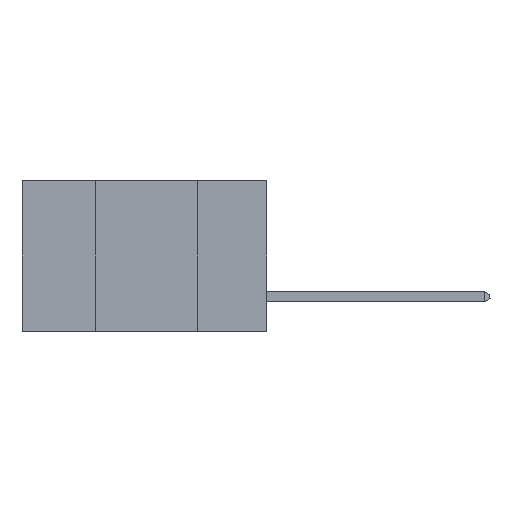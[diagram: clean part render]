
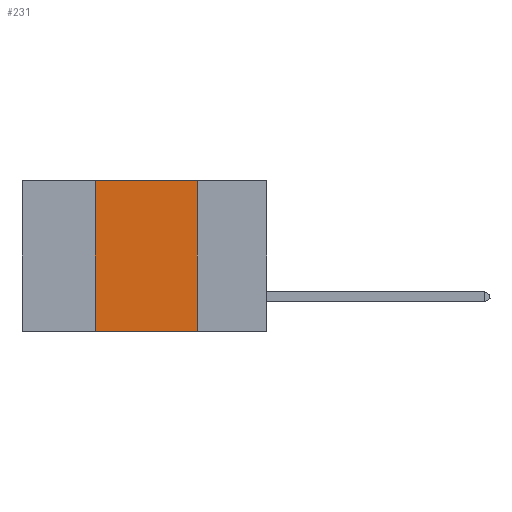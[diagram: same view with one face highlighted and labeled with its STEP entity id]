
A CAD part, left-side view. The second image highlights one B-rep face of the part: STEP entity #231.
In plain terms, the highlighted planar face has unit normal (-1, 0, 0).
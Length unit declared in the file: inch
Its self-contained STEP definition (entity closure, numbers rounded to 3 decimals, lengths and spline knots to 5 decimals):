
#231 = ADVANCED_FACE ( 'NONE', ( #3089 ), #13129, .F. ) ;
#276 = AXIS2_PLACEMENT_3D ( 'NONE', #3503, #13479, #14699 ) ;
#319 = EDGE_LOOP ( 'NONE', ( #8522, #7369, #3352, #14893 ) ) ;
#569 = LINE ( 'NONE', #1168, #6791 ) ;
#681 = CARTESIAN_POINT ( 'NONE',  ( 0., 0.42, -0.37 ) ) ;
#1168 = CARTESIAN_POINT ( 'NONE',  ( 0., 0.42, 0. ) ) ;
#1936 = VECTOR ( 'NONE', #8926, 39.37008 ) ;
#2264 = EDGE_CURVE ( 'NONE', #6485, #10681, #14938, .T. ) ;
#2975 = DIRECTION ( 'NONE',  ( 0., -1., 0. ) ) ;
#3089 = FACE_OUTER_BOUND ( 'NONE', #319, .T. ) ;
#3352 = ORIENTED_EDGE ( 'NONE', *, *, #12918, .F. ) ;
#3503 = CARTESIAN_POINT ( 'NONE',  ( 0., 0.6, 0. ) ) ;
#5904 = CARTESIAN_POINT ( 'NONE',  ( 0., 0.17, 0. ) ) ;
#6341 = LINE ( 'NONE', #9029, #12589 ) ;
#6411 = CARTESIAN_POINT ( 'NONE',  ( 0., 0.6, -0.37 ) ) ;
#6485 = VERTEX_POINT ( 'NONE', #5904 ) ;
#6791 = VECTOR ( 'NONE', #10845, 39.37008 ) ;
#7369 = ORIENTED_EDGE ( 'NONE', *, *, #9135, .F. ) ;
#7451 = LINE ( 'NONE', #6411, #1936 ) ;
#8522 = ORIENTED_EDGE ( 'NONE', *, *, #2264, .F. ) ;
#8711 = CARTESIAN_POINT ( 'NONE',  ( 0., 0.42, 0. ) ) ;
#8923 = VERTEX_POINT ( 'NONE', #8711 ) ;
#8926 = DIRECTION ( 'NONE',  ( 0., -1., 0. ) ) ;
#9029 = CARTESIAN_POINT ( 'NONE',  ( 0., 0.6, 0. ) ) ;
#9135 = EDGE_CURVE ( 'NONE', #8923, #6485, #6341, .T. ) ;
#10681 = VERTEX_POINT ( 'NONE', #13381 ) ;
#10845 = DIRECTION ( 'NONE',  ( 0., 0., 1. ) ) ;
#11028 = EDGE_CURVE ( 'NONE', #11249, #10681, #7451, .T. ) ;
#11249 = VERTEX_POINT ( 'NONE', #681 ) ;
#11532 = VECTOR ( 'NONE', #15132, 39.37008 ) ;
#12589 = VECTOR ( 'NONE', #2975, 39.37008 ) ;
#12801 = CARTESIAN_POINT ( 'NONE',  ( 0., 0.17, 0. ) ) ;
#12918 = EDGE_CURVE ( 'NONE', #11249, #8923, #569, .T. ) ;
#13129 = PLANE ( 'NONE',  #276 ) ;
#13381 = CARTESIAN_POINT ( 'NONE',  ( 0., 0.17, -0.37 ) ) ;
#13479 = DIRECTION ( 'NONE',  ( 1., 0., 0. ) ) ;
#14699 = DIRECTION ( 'NONE',  ( 0., 0., -1. ) ) ;
#14893 = ORIENTED_EDGE ( 'NONE', *, *, #11028, .T. ) ;
#14938 = LINE ( 'NONE', #12801, #11532 ) ;
#15132 = DIRECTION ( 'NONE',  ( 0., 0., -1. ) ) ;
